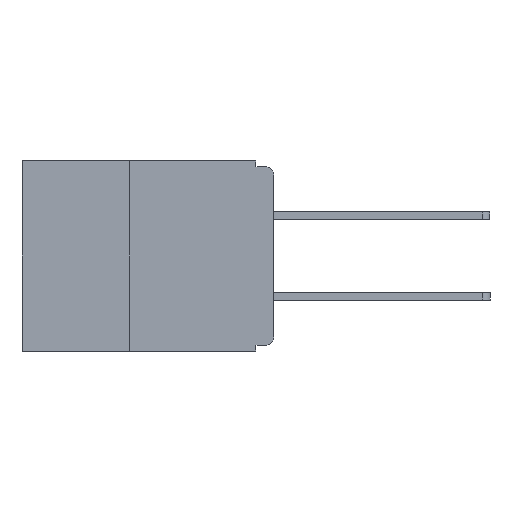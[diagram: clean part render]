
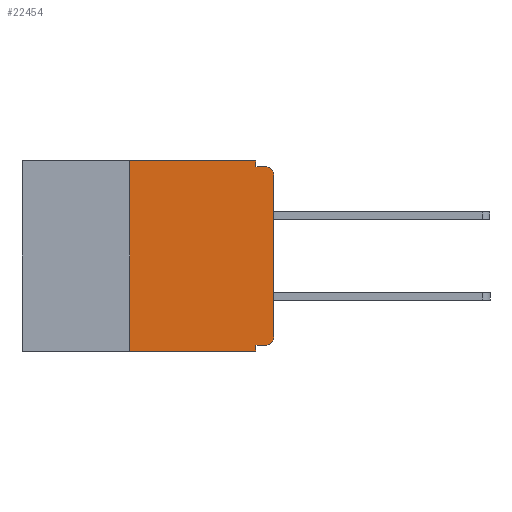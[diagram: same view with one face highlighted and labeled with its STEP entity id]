
A CAD part, left-side view. The second image highlights one B-rep face of the part: STEP entity #22454.
In plain terms, the highlighted planar face has unit normal (-1, 0, 0).
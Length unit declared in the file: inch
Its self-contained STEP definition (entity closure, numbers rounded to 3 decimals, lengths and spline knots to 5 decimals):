
#241 = PLANE ( 'NONE',  #2984 ) ;
#1005 = EDGE_CURVE ( 'NONE', #14849, #25167, #26559, .T. ) ;
#1587 = EDGE_CURVE ( 'NONE', #28625, #11306, #31467, .T. ) ;
#1717 = CARTESIAN_POINT ( 'NONE',  ( 0., 0.015, -0.32 ) ) ;
#2145 = CARTESIAN_POINT ( 'NONE',  ( 0., 0.437, 0. ) ) ;
#2284 = EDGE_CURVE ( 'NONE', #29990, #4883, #3412, .T. ) ;
#2375 = ORIENTED_EDGE ( 'NONE', *, *, #1587, .F. ) ;
#2825 = DIRECTION ( 'NONE',  ( 1., 0., 0. ) ) ;
#2984 = AXIS2_PLACEMENT_3D ( 'NONE', #18109, #2825, #20664 ) ;
#3033 = LINE ( 'NONE', #23279, #15000 ) ;
#3207 = CARTESIAN_POINT ( 'NONE',  ( 0., 0., -0.32 ) ) ;
#3412 = LINE ( 'NONE', #31513, #29535 ) ;
#3461 = CARTESIAN_POINT ( 'NONE',  ( 0., 0., -0.305 ) ) ;
#3979 = ORIENTED_EDGE ( 'NONE', *, *, #1005, .T. ) ;
#3987 = AXIS2_PLACEMENT_3D ( 'NONE', #22221, #7014, #24763 ) ;
#4319 = VECTOR ( 'NONE', #30330, 39.37008 ) ;
#4808 = DIRECTION ( 'NONE',  ( 0., 0., -1. ) ) ;
#4883 = VERTEX_POINT ( 'NONE', #10839 ) ;
#5577 = CARTESIAN_POINT ( 'NONE',  ( 0., 0.031, 0. ) ) ;
#5659 = EDGE_CURVE ( 'NONE', #25167, #23988, #6731, .T. ) ;
#5827 = DIRECTION ( 'NONE',  ( 0., 1., 0. ) ) ;
#6493 = DIRECTION ( 'NONE',  ( -1., 0., 0. ) ) ;
#6496 = EDGE_CURVE ( 'NONE', #14153, #13232, #10304, .T. ) ;
#6637 = FACE_OUTER_BOUND ( 'NONE', #20054, .T. ) ;
#6731 = CIRCLE ( 'NONE', #9832, 0.015 ) ;
#7014 = DIRECTION ( 'NONE',  ( -1., 0., 0. ) ) ;
#7236 = EDGE_CURVE ( 'NONE', #11306, #23988, #3033, .T. ) ;
#7809 = ORIENTED_EDGE ( 'NONE', *, *, #6496, .F. ) ;
#8988 = LINE ( 'NONE', #9092, #23288 ) ;
#9092 = CARTESIAN_POINT ( 'NONE',  ( 0., 0.437, -0.33 ) ) ;
#9832 = AXIS2_PLACEMENT_3D ( 'NONE', #21672, #6493, #24240 ) ;
#10304 = LINE ( 'NONE', #12744, #4319 ) ;
#10839 = CARTESIAN_POINT ( 'NONE',  ( 0., 0.25, 0. ) ) ;
#11292 = ORIENTED_EDGE ( 'NONE', *, *, #2284, .F. ) ;
#11306 = VERTEX_POINT ( 'NONE', #17749 ) ;
#12269 = CARTESIAN_POINT ( 'NONE',  ( 0., 0.031, -0.33 ) ) ;
#12299 = VECTOR ( 'NONE', #19722, 39.37008 ) ;
#12744 = CARTESIAN_POINT ( 'NONE',  ( 0., 0.031, -0.33 ) ) ;
#13232 = VERTEX_POINT ( 'NONE', #12269 ) ;
#13256 = LINE ( 'NONE', #3207, #19258 ) ;
#13751 = CARTESIAN_POINT ( 'NONE',  ( 0., 0.031, -0.32 ) ) ;
#13812 = EDGE_CURVE ( 'NONE', #22128, #14849, #17773, .T. ) ;
#14153 = VERTEX_POINT ( 'NONE', #13751 ) ;
#14458 = CARTESIAN_POINT ( 'NONE',  ( 0., 0.25, -0.33 ) ) ;
#14849 = VERTEX_POINT ( 'NONE', #3461 ) ;
#14862 = DIRECTION ( 'NONE',  ( 0., -1., 0. ) ) ;
#14935 = EDGE_CURVE ( 'NONE', #29990, #13232, #8988, .T. ) ;
#15000 = VECTOR ( 'NONE', #25773, 39.37008 ) ;
#16600 = VECTOR ( 'NONE', #4808, 39.37008 ) ;
#17749 = CARTESIAN_POINT ( 'NONE',  ( 0., 0.031, -0.01 ) ) ;
#17773 = CIRCLE ( 'NONE', #3987, 0.015 ) ;
#18109 = CARTESIAN_POINT ( 'NONE',  ( 0., 0.437, 0. ) ) ;
#19258 = VECTOR ( 'NONE', #5827, 39.37008 ) ;
#19572 = CARTESIAN_POINT ( 'NONE',  ( 0., 0.015, -0.01 ) ) ;
#19654 = CARTESIAN_POINT ( 'NONE',  ( 0., 0., 0. ) ) ;
#19722 = DIRECTION ( 'NONE',  ( 0., 0., 1. ) ) ;
#20054 = EDGE_LOOP ( 'NONE', ( #3979, #27451, #24839, #2375, #27021, #11292, #22119, #7809, #26161, #20100 ) ) ;
#20100 = ORIENTED_EDGE ( 'NONE', *, *, #13812, .T. ) ;
#20262 = CARTESIAN_POINT ( 'NONE',  ( 0., 0., -0.025 ) ) ;
#20664 = DIRECTION ( 'NONE',  ( 0., 0., -1. ) ) ;
#21672 = CARTESIAN_POINT ( 'NONE',  ( 0., 0.015, -0.025 ) ) ;
#21847 = EDGE_CURVE ( 'NONE', #22128, #14153, #13256, .T. ) ;
#22119 = ORIENTED_EDGE ( 'NONE', *, *, #14935, .T. ) ;
#22128 = VERTEX_POINT ( 'NONE', #1717 ) ;
#22221 = CARTESIAN_POINT ( 'NONE',  ( 0., 0.015, -0.305 ) ) ;
#22454 = ADVANCED_FACE ( 'NONE', ( #6637 ), #241, .F. ) ;
#23279 = CARTESIAN_POINT ( 'NONE',  ( 0., 0., -0.01 ) ) ;
#23288 = VECTOR ( 'NONE', #29238, 39.37008 ) ;
#23908 = CARTESIAN_POINT ( 'NONE',  ( 0., 0.031, 0. ) ) ;
#23988 = VERTEX_POINT ( 'NONE', #19572 ) ;
#24240 = DIRECTION ( 'NONE',  ( 0., 0., -1. ) ) ;
#24763 = DIRECTION ( 'NONE',  ( 0., 0., -1. ) ) ;
#24839 = ORIENTED_EDGE ( 'NONE', *, *, #7236, .F. ) ;
#25167 = VERTEX_POINT ( 'NONE', #20262 ) ;
#25773 = DIRECTION ( 'NONE',  ( 0., -1., 0. ) ) ;
#26161 = ORIENTED_EDGE ( 'NONE', *, *, #21847, .F. ) ;
#26345 = VECTOR ( 'NONE', #14862, 39.37008 ) ;
#26559 = LINE ( 'NONE', #19654, #12299 ) ;
#27021 = ORIENTED_EDGE ( 'NONE', *, *, #31464, .F. ) ;
#27123 = LINE ( 'NONE', #2145, #26345 ) ;
#27451 = ORIENTED_EDGE ( 'NONE', *, *, #5659, .T. ) ;
#28625 = VERTEX_POINT ( 'NONE', #23908 ) ;
#29238 = DIRECTION ( 'NONE',  ( 0., -1., 0. ) ) ;
#29535 = VECTOR ( 'NONE', #31171, 39.37008 ) ;
#29990 = VERTEX_POINT ( 'NONE', #14458 ) ;
#30330 = DIRECTION ( 'NONE',  ( 0., 0., -1. ) ) ;
#31171 = DIRECTION ( 'NONE',  ( 0., 0., 1. ) ) ;
#31464 = EDGE_CURVE ( 'NONE', #4883, #28625, #27123, .T. ) ;
#31467 = LINE ( 'NONE', #5577, #16600 ) ;
#31513 = CARTESIAN_POINT ( 'NONE',  ( 0., 0.25, -0.33 ) ) ;
